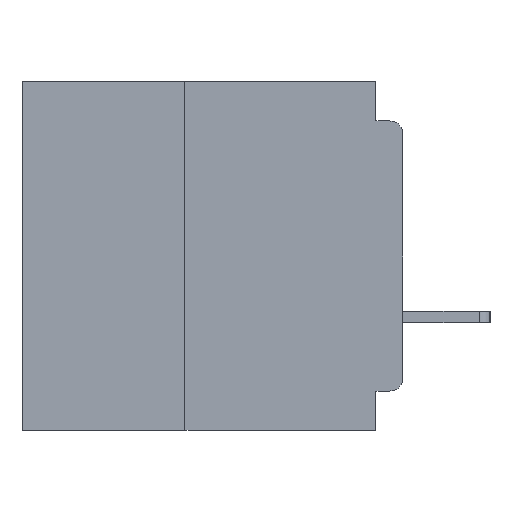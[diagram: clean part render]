
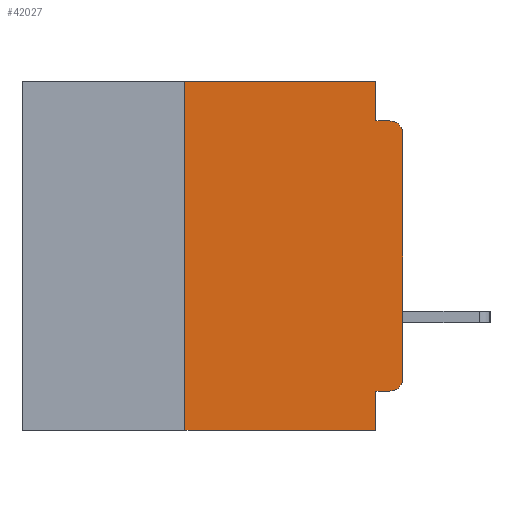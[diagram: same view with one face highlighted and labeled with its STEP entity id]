
A CAD part, left-side view. The second image highlights one B-rep face of the part: STEP entity #42027.
In plain terms, the highlighted planar face has unit normal (-1, 0, 0).
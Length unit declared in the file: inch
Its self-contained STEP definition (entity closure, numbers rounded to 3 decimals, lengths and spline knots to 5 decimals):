
#621 = ORIENTED_EDGE ( 'NONE', *, *, #39500, .F. ) ;
#1247 = VECTOR ( 'NONE', #25043, 39.37008 ) ;
#1910 = LINE ( 'NONE', #28777, #49732 ) ;
#1919 = LINE ( 'NONE', #8215, #45558 ) ;
#2026 = CARTESIAN_POINT ( 'NONE',  ( 0., 0., -0.34 ) ) ;
#2080 = VERTEX_POINT ( 'NONE', #5398 ) ;
#3542 = VECTOR ( 'NONE', #27131, 39.37008 ) ;
#4544 = LINE ( 'NONE', #9705, #50893 ) ;
#4847 = VERTEX_POINT ( 'NONE', #19626 ) ;
#4950 = LINE ( 'NONE', #36150, #3542 ) ;
#5398 = CARTESIAN_POINT ( 'NONE',  ( 0., 0.25, -0.4 ) ) ;
#6469 = CARTESIAN_POINT ( 'NONE',  ( 0., 0., -0.045 ) ) ;
#7465 = DIRECTION ( 'NONE',  ( 0., 1., 0. ) ) ;
#7701 = ORIENTED_EDGE ( 'NONE', *, *, #17093, .F. ) ;
#8137 = CIRCLE ( 'NONE', #44467, 0.015 ) ;
#8215 = CARTESIAN_POINT ( 'NONE',  ( 0., 0., 0. ) ) ;
#8439 = VECTOR ( 'NONE', #7465, 39.37008 ) ;
#8647 = CARTESIAN_POINT ( 'NONE',  ( 0., 0.015, -0.06 ) ) ;
#8947 = AXIS2_PLACEMENT_3D ( 'NONE', #46394, #19553, #50826 ) ;
#9705 = CARTESIAN_POINT ( 'NONE',  ( 0., 0.437, 0. ) ) ;
#10735 = DIRECTION ( 'NONE',  ( 0., 0., -1. ) ) ;
#10981 = DIRECTION ( 'NONE',  ( 0., -1., 0. ) ) ;
#11471 = EDGE_CURVE ( 'NONE', #4847, #28304, #8137, .T. ) ;
#11494 = CARTESIAN_POINT ( 'NONE',  ( 0., 0.031, 0. ) ) ;
#12213 = CARTESIAN_POINT ( 'NONE',  ( 0., 0.437, -0.4 ) ) ;
#12804 = EDGE_CURVE ( 'NONE', #36190, #16084, #4544, .T. ) ;
#13211 = DIRECTION ( 'NONE',  ( 0., 0., -1. ) ) ;
#13361 = ORIENTED_EDGE ( 'NONE', *, *, #20686, .F. ) ;
#14092 = LINE ( 'NONE', #6469, #36687 ) ;
#14712 = LINE ( 'NONE', #11494, #1247 ) ;
#15545 = VECTOR ( 'NONE', #43693, 39.37008 ) ;
#15828 = VERTEX_POINT ( 'NONE', #38486 ) ;
#16084 = VERTEX_POINT ( 'NONE', #49147 ) ;
#16411 = EDGE_CURVE ( 'NONE', #15828, #28304, #14092, .T. ) ;
#17093 = EDGE_CURVE ( 'NONE', #16084, #15828, #14712, .T. ) ;
#17193 = CARTESIAN_POINT ( 'NONE',  ( 0., 0.25, 0. ) ) ;
#18001 = CIRCLE ( 'NONE', #8947, 0.015 ) ;
#18902 = CARTESIAN_POINT ( 'NONE',  ( 0., 0.437, 0. ) ) ;
#19075 = ORIENTED_EDGE ( 'NONE', *, *, #29660, .F. ) ;
#19291 = AXIS2_PLACEMENT_3D ( 'NONE', #18902, #23496, #54656 ) ;
#19553 = DIRECTION ( 'NONE',  ( -1., 0., 0. ) ) ;
#19626 = CARTESIAN_POINT ( 'NONE',  ( 0., 0., -0.06 ) ) ;
#20686 = EDGE_CURVE ( 'NONE', #2080, #36190, #4950, .T. ) ;
#21940 = DIRECTION ( 'NONE',  ( 0., 0., 1. ) ) ;
#23392 = LINE ( 'NONE', #52197, #8439 ) ;
#23408 = VERTEX_POINT ( 'NONE', #45221 ) ;
#23496 = DIRECTION ( 'NONE',  ( 1., 0., 0. ) ) ;
#25043 = DIRECTION ( 'NONE',  ( 0., 0., -1. ) ) ;
#25046 = EDGE_CURVE ( 'NONE', #2080, #23408, #27598, .T. ) ;
#25672 = CARTESIAN_POINT ( 'NONE',  ( 0., 0.031, -0.355 ) ) ;
#26163 = ORIENTED_EDGE ( 'NONE', *, *, #11471, .T. ) ;
#27131 = DIRECTION ( 'NONE',  ( 0., 0., 1. ) ) ;
#27598 = LINE ( 'NONE', #12213, #15545 ) ;
#27768 = VERTEX_POINT ( 'NONE', #2026 ) ;
#28304 = VERTEX_POINT ( 'NONE', #55718 ) ;
#28777 = CARTESIAN_POINT ( 'NONE',  ( 0., 0.031, -0.4 ) ) ;
#29660 = EDGE_CURVE ( 'NONE', #40084, #23408, #1910, .T. ) ;
#31947 = EDGE_CURVE ( 'NONE', #35904, #27768, #18001, .T. ) ;
#35904 = VERTEX_POINT ( 'NONE', #41957 ) ;
#35979 = ORIENTED_EDGE ( 'NONE', *, *, #12804, .F. ) ;
#36150 = CARTESIAN_POINT ( 'NONE',  ( 0., 0.25, -0.4 ) ) ;
#36190 = VERTEX_POINT ( 'NONE', #17193 ) ;
#36687 = VECTOR ( 'NONE', #10981, 39.37008 ) ;
#36706 = ORIENTED_EDGE ( 'NONE', *, *, #31947, .T. ) ;
#38486 = CARTESIAN_POINT ( 'NONE',  ( 0., 0.031, -0.045 ) ) ;
#39500 = EDGE_CURVE ( 'NONE', #35904, #40084, #23392, .T. ) ;
#40084 = VERTEX_POINT ( 'NONE', #25672 ) ;
#40198 = DIRECTION ( 'NONE',  ( -1., 0., 0. ) ) ;
#41957 = CARTESIAN_POINT ( 'NONE',  ( 0., 0.015, -0.355 ) ) ;
#42027 = ADVANCED_FACE ( 'NONE', ( #52470 ), #45748, .F. ) ;
#42214 = ORIENTED_EDGE ( 'NONE', *, *, #16411, .F. ) ;
#43693 = DIRECTION ( 'NONE',  ( 0., -1., 0. ) ) ;
#44467 = AXIS2_PLACEMENT_3D ( 'NONE', #8647, #40198, #13211 ) ;
#45221 = CARTESIAN_POINT ( 'NONE',  ( 0., 0.031, -0.4 ) ) ;
#45558 = VECTOR ( 'NONE', #21940, 39.37008 ) ;
#45748 = PLANE ( 'NONE',  #19291 ) ;
#46394 = CARTESIAN_POINT ( 'NONE',  ( 0., 0.015, -0.34 ) ) ;
#48486 = ORIENTED_EDGE ( 'NONE', *, *, #52758, .T. ) ;
#49147 = CARTESIAN_POINT ( 'NONE',  ( 0., 0.031, 0. ) ) ;
#49195 = ORIENTED_EDGE ( 'NONE', *, *, #25046, .T. ) ;
#49732 = VECTOR ( 'NONE', #10735, 39.37008 ) ;
#50170 = DIRECTION ( 'NONE',  ( 0., -1., 0. ) ) ;
#50826 = DIRECTION ( 'NONE',  ( 0., 0., -1. ) ) ;
#50893 = VECTOR ( 'NONE', #50170, 39.37008 ) ;
#52197 = CARTESIAN_POINT ( 'NONE',  ( 0., 0., -0.355 ) ) ;
#52470 = FACE_OUTER_BOUND ( 'NONE', #54768, .T. ) ;
#52758 = EDGE_CURVE ( 'NONE', #27768, #4847, #1919, .T. ) ;
#54656 = DIRECTION ( 'NONE',  ( 0., 0., -1. ) ) ;
#54768 = EDGE_LOOP ( 'NONE', ( #48486, #26163, #42214, #7701, #35979, #13361, #49195, #19075, #621, #36706 ) ) ;
#55718 = CARTESIAN_POINT ( 'NONE',  ( 0., 0.015, -0.045 ) ) ;
